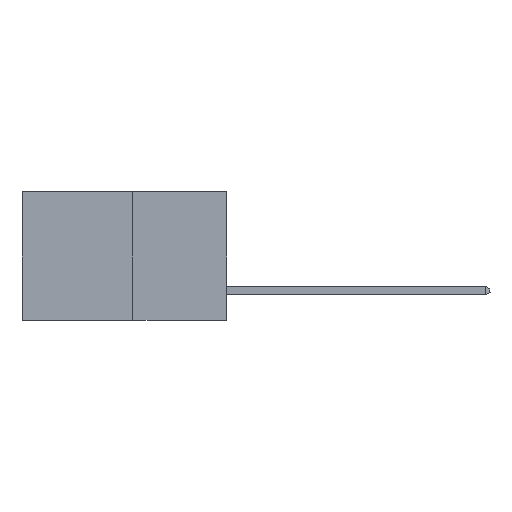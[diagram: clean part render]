
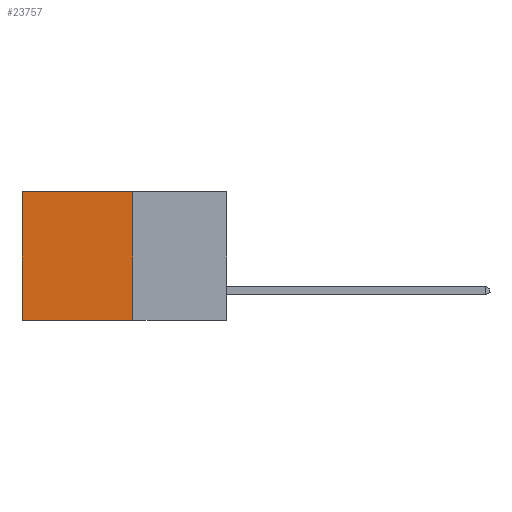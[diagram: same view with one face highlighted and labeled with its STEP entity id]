
A CAD part, left-side view. The second image highlights one B-rep face of the part: STEP entity #23757.
In plain terms, the highlighted planar face has unit normal (-1, 0, 0).
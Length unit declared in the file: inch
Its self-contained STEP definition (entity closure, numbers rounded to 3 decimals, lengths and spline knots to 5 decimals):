
#3 = PLANE ( 'NONE',  #23310 ) ;
#1582 = ORIENTED_EDGE ( 'NONE', *, *, #20858, .F. ) ;
#1652 = VECTOR ( 'NONE', #30637, 39.37008 ) ;
#1831 = EDGE_CURVE ( 'NONE', #22582, #11196, #21087, .T. ) ;
#2420 = CARTESIAN_POINT ( 'NONE',  ( 0.277, 0.27, -0.37 ) ) ;
#3567 = CARTESIAN_POINT ( 'NONE',  ( 0.277, 0.59, -0.37 ) ) ;
#3933 = DIRECTION ( 'NONE',  ( 0., 1., 0. ) ) ;
#3992 = EDGE_LOOP ( 'NONE', ( #16360, #1582, #11135, #25009 ) ) ;
#4822 = EDGE_CURVE ( 'NONE', #7740, #7297, #20133, .T. ) ;
#4831 = DIRECTION ( 'NONE',  ( 0., 0., -1. ) ) ;
#7142 = LINE ( 'NONE', #8726, #19361 ) ;
#7297 = VERTEX_POINT ( 'NONE', #27089 ) ;
#7740 = VERTEX_POINT ( 'NONE', #21379 ) ;
#8726 = CARTESIAN_POINT ( 'NONE',  ( 0.277, 0.27, 0. ) ) ;
#11135 = ORIENTED_EDGE ( 'NONE', *, *, #4822, .F. ) ;
#11196 = VERTEX_POINT ( 'NONE', #3567 ) ;
#13649 = VECTOR ( 'NONE', #21817, 39.37008 ) ;
#16040 = CARTESIAN_POINT ( 'NONE',  ( 0.277, 0.27, -0.37 ) ) ;
#16360 = ORIENTED_EDGE ( 'NONE', *, *, #1831, .T. ) ;
#16780 = LINE ( 'NONE', #28393, #28870 ) ;
#19361 = VECTOR ( 'NONE', #3933, 39.37008 ) ;
#19454 = DIRECTION ( 'NONE',  ( 1., 0., 0. ) ) ;
#19846 = CARTESIAN_POINT ( 'NONE',  ( 0.277, 0.59, 0. ) ) ;
#20133 = LINE ( 'NONE', #16040, #13649 ) ;
#20858 = EDGE_CURVE ( 'NONE', #7297, #11196, #16780, .T. ) ;
#21087 = LINE ( 'NONE', #27531, #1652 ) ;
#21258 = DIRECTION ( 'NONE',  ( 0., 1., 0. ) ) ;
#21379 = CARTESIAN_POINT ( 'NONE',  ( 0.277, 0.27, 0. ) ) ;
#21817 = DIRECTION ( 'NONE',  ( 0., 0., -1. ) ) ;
#22582 = VERTEX_POINT ( 'NONE', #19846 ) ;
#23310 = AXIS2_PLACEMENT_3D ( 'NONE', #2420, #19454, #4831 ) ;
#23757 = ADVANCED_FACE ( 'NONE', ( #30686 ), #3, .F. ) ;
#25009 = ORIENTED_EDGE ( 'NONE', *, *, #25218, .T. ) ;
#25218 = EDGE_CURVE ( 'NONE', #7740, #22582, #7142, .T. ) ;
#27089 = CARTESIAN_POINT ( 'NONE',  ( 0.277, 0.27, -0.37 ) ) ;
#27531 = CARTESIAN_POINT ( 'NONE',  ( 0.277, 0.59, -0.37 ) ) ;
#28393 = CARTESIAN_POINT ( 'NONE',  ( 0.277, 0.27, -0.37 ) ) ;
#28870 = VECTOR ( 'NONE', #21258, 39.37008 ) ;
#30637 = DIRECTION ( 'NONE',  ( 0., 0., -1. ) ) ;
#30686 = FACE_OUTER_BOUND ( 'NONE', #3992, .T. ) ;
